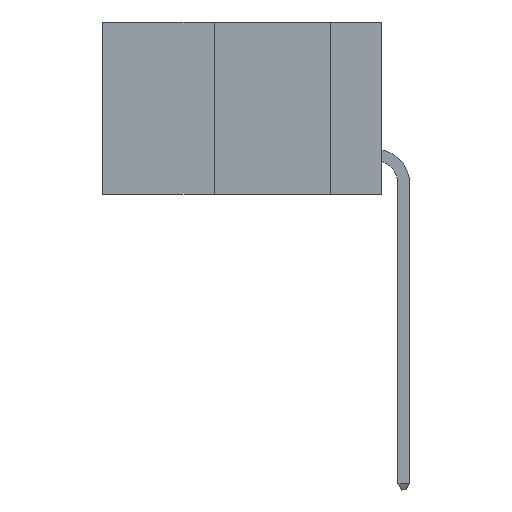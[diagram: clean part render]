
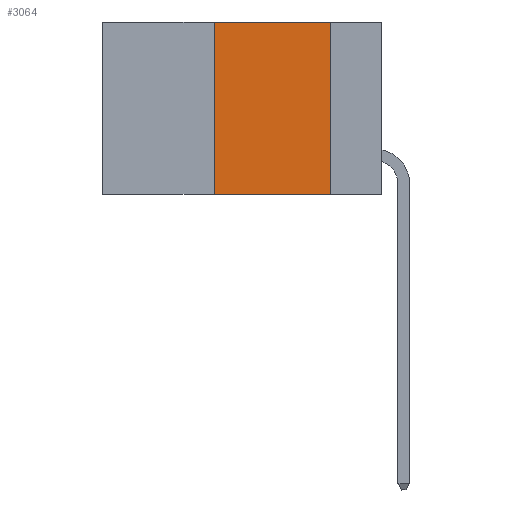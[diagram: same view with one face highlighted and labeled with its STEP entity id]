
A CAD part, left-side view. The second image highlights one B-rep face of the part: STEP entity #3064.
In plain terms, the highlighted planar face has unit normal (-1, 0, 0).
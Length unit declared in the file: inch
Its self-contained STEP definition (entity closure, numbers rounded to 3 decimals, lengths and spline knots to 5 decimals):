
#203 = EDGE_CURVE ( 'NONE', #3675, #6597, #263, .T. ) ;
#263 = LINE ( 'NONE', #1741, #7409 ) ;
#454 = ORIENTED_EDGE ( 'NONE', *, *, #4859, .T. ) ;
#669 = CARTESIAN_POINT ( 'NONE',  ( 0., 0.36, 0. ) ) ;
#706 = DIRECTION ( 'NONE',  ( 1., 0., 0. ) ) ;
#957 = LINE ( 'NONE', #4118, #8571 ) ;
#1451 = CARTESIAN_POINT ( 'NONE',  ( 0., 0.36, -0.37 ) ) ;
#1484 = FACE_OUTER_BOUND ( 'NONE', #4009, .T. ) ;
#1737 = DIRECTION ( 'NONE',  ( 0., -1., 0. ) ) ;
#1741 = CARTESIAN_POINT ( 'NONE',  ( 0., 0.11, 0. ) ) ;
#2024 = CARTESIAN_POINT ( 'NONE',  ( 0., 0.11, 0. ) ) ;
#2111 = VERTEX_POINT ( 'NONE', #1451 ) ;
#2331 = CARTESIAN_POINT ( 'NONE',  ( 0., 0.6, 0. ) ) ;
#2747 = CARTESIAN_POINT ( 'NONE',  ( 0., 0.6, 0. ) ) ;
#3064 = ADVANCED_FACE ( 'NONE', ( #1484 ), #4695, .F. ) ;
#3675 = VERTEX_POINT ( 'NONE', #2024 ) ;
#3728 = EDGE_CURVE ( 'NONE', #9950, #3675, #8984, .T. ) ;
#4009 = EDGE_LOOP ( 'NONE', ( #8956, #4318, #4067, #454 ) ) ;
#4067 = ORIENTED_EDGE ( 'NONE', *, *, #9124, .F. ) ;
#4118 = CARTESIAN_POINT ( 'NONE',  ( 0., 0.6, -0.37 ) ) ;
#4318 = ORIENTED_EDGE ( 'NONE', *, *, #3728, .F. ) ;
#4340 = DIRECTION ( 'NONE',  ( 0., -1., 0. ) ) ;
#4695 = PLANE ( 'NONE',  #8542 ) ;
#4859 = EDGE_CURVE ( 'NONE', #2111, #6597, #957, .T. ) ;
#5277 = VECTOR ( 'NONE', #5865, 39.37008 ) ;
#5780 = CARTESIAN_POINT ( 'NONE',  ( 0., 0.11, -0.37 ) ) ;
#5865 = DIRECTION ( 'NONE',  ( 0., 0., 1. ) ) ;
#6529 = CARTESIAN_POINT ( 'NONE',  ( 0., 0.36, 0. ) ) ;
#6597 = VERTEX_POINT ( 'NONE', #5780 ) ;
#6909 = VECTOR ( 'NONE', #4340, 39.37008 ) ;
#7125 = LINE ( 'NONE', #6529, #5277 ) ;
#7409 = VECTOR ( 'NONE', #9485, 39.37008 ) ;
#8542 = AXIS2_PLACEMENT_3D ( 'NONE', #2331, #706, #9404 ) ;
#8571 = VECTOR ( 'NONE', #1737, 39.37008 ) ;
#8956 = ORIENTED_EDGE ( 'NONE', *, *, #203, .F. ) ;
#8984 = LINE ( 'NONE', #2747, #6909 ) ;
#9124 = EDGE_CURVE ( 'NONE', #2111, #9950, #7125, .T. ) ;
#9404 = DIRECTION ( 'NONE',  ( 0., 0., -1. ) ) ;
#9485 = DIRECTION ( 'NONE',  ( 0., 0., -1. ) ) ;
#9950 = VERTEX_POINT ( 'NONE', #669 ) ;
